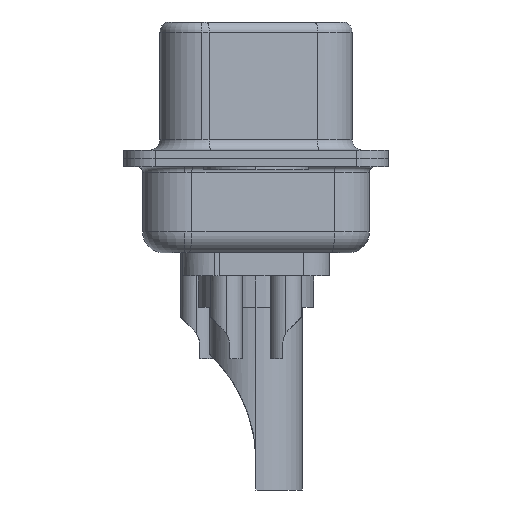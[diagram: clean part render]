
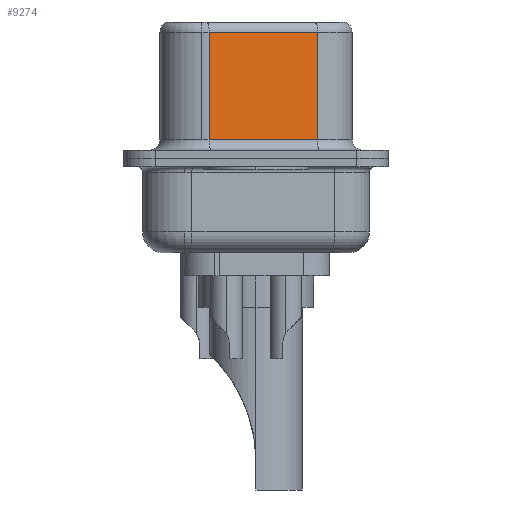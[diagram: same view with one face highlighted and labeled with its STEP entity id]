
A CAD part, left-side view. The second image highlights one B-rep face of the part: STEP entity #9274.
In plain terms, the highlighted planar face has unit normal (-0.985, -0.174, 0).
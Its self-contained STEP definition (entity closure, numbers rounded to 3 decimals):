
#92 = CARTESIAN_POINT ( 'NONE',  ( 4.585, -2.927, 0.9 ) ) ;
#376 = DIRECTION ( 'NONE',  ( 0., 0., -1. ) ) ;
#1055 = VERTEX_POINT ( 'NONE', #4699 ) ;
#1474 = DIRECTION ( 'NONE',  ( -0.174, 0.985, 0. ) ) ;
#2042 = VECTOR ( 'NONE', #11769, 1000. ) ;
#2060 = CARTESIAN_POINT ( 'NONE',  ( 4.585, -2.927, 6.52 ) ) ;
#2894 = PLANE ( 'NONE',  #16207 ) ;
#3035 = CARTESIAN_POINT ( 'NONE',  ( 4.585, -2.927, 6.02 ) ) ;
#3075 = ORIENTED_EDGE ( 'NONE', *, *, #4549, .T. ) ;
#3377 = CARTESIAN_POINT ( 'NONE',  ( 4.585, -2.927, 0.9 ) ) ;
#3926 = VERTEX_POINT ( 'NONE', #3377 ) ;
#4079 = EDGE_LOOP ( 'NONE', ( #7819, #18149, #3075, #9159 ) ) ;
#4549 = EDGE_CURVE ( 'NONE', #6735, #1055, #8298, .T. ) ;
#4699 = CARTESIAN_POINT ( 'NONE',  ( 3.675, 2.233, 0.9 ) ) ;
#5788 = LINE ( 'NONE', #92, #16891 ) ;
#6010 = DIRECTION ( 'NONE',  ( 0.174, -0.985, 0. ) ) ;
#6735 = VERTEX_POINT ( 'NONE', #18370 ) ;
#6895 = LINE ( 'NONE', #11588, #15683 ) ;
#7449 = CARTESIAN_POINT ( 'NONE',  ( 3.675, 2.233, 6.52 ) ) ;
#7819 = ORIENTED_EDGE ( 'NONE', *, *, #11713, .F. ) ;
#8298 = LINE ( 'NONE', #7449, #2042 ) ;
#9042 = VERTEX_POINT ( 'NONE', #3035 ) ;
#9159 = ORIENTED_EDGE ( 'NONE', *, *, #9970, .T. ) ;
#9274 = ADVANCED_FACE ( 'NONE', ( #18074 ), #2894, .F. ) ;
#9970 = EDGE_CURVE ( 'NONE', #1055, #3926, #5788, .T. ) ;
#10207 = DIRECTION ( 'NONE',  ( -0.174, 0.985, 0. ) ) ;
#11588 = CARTESIAN_POINT ( 'NONE',  ( 4.585, -2.927, 6.02 ) ) ;
#11713 = EDGE_CURVE ( 'NONE', #9042, #3926, #16510, .T. ) ;
#11769 = DIRECTION ( 'NONE',  ( 0., 0., -1. ) ) ;
#11858 = CARTESIAN_POINT ( 'NONE',  ( 4.585, -2.927, 6.52 ) ) ;
#14875 = VECTOR ( 'NONE', #376, 1000. ) ;
#15683 = VECTOR ( 'NONE', #10207, 1000. ) ;
#16207 = AXIS2_PLACEMENT_3D ( 'NONE', #11858, #19056, #1474 ) ;
#16510 = LINE ( 'NONE', #2060, #14875 ) ;
#16666 = EDGE_CURVE ( 'NONE', #9042, #6735, #6895, .T. ) ;
#16891 = VECTOR ( 'NONE', #6010, 1000. ) ;
#18074 = FACE_OUTER_BOUND ( 'NONE', #4079, .T. ) ;
#18149 = ORIENTED_EDGE ( 'NONE', *, *, #16666, .T. ) ;
#18370 = CARTESIAN_POINT ( 'NONE',  ( 3.675, 2.233, 6.02 ) ) ;
#19056 = DIRECTION ( 'NONE',  ( 0.985, 0.174, 0. ) ) ;
